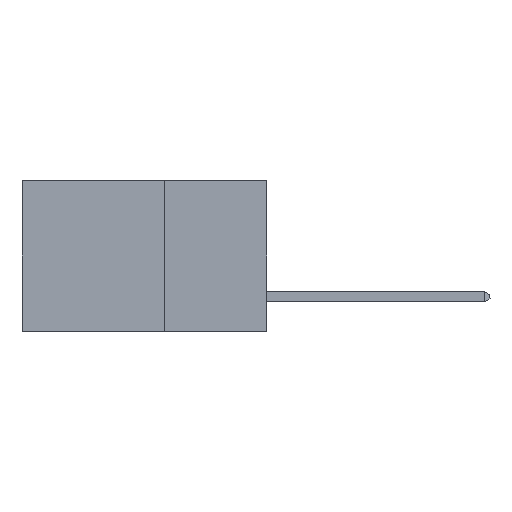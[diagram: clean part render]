
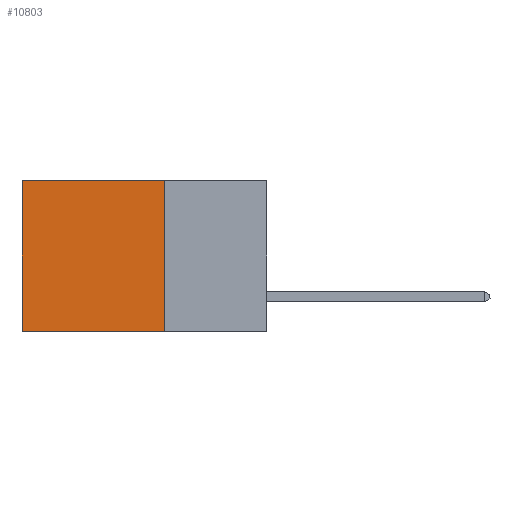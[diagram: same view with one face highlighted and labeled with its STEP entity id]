
A CAD part, left-side view. The second image highlights one B-rep face of the part: STEP entity #10803.
In plain terms, the highlighted planar face has unit normal (-1, 0, 0).
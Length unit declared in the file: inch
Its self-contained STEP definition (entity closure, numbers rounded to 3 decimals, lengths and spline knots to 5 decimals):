
#1214 = DIRECTION ( 'NONE',  ( 1., 0., 0. ) ) ;
#2312 = DIRECTION ( 'NONE',  ( 0., 0., -1. ) ) ;
#2350 = DIRECTION ( 'NONE',  ( 0., 1., 0. ) ) ;
#3029 = ORIENTED_EDGE ( 'NONE', *, *, #13267, .T. ) ;
#4931 = PLANE ( 'NONE',  #16104 ) ;
#4991 = LINE ( 'NONE', #15347, #39008 ) ;
#9588 = VECTOR ( 'NONE', #19865, 39.37008 ) ;
#10803 = ADVANCED_FACE ( 'NONE', ( #30011 ), #4931, .F. ) ;
#11649 = CARTESIAN_POINT ( 'NONE',  ( 0.2875, 0.25, 0. ) ) ;
#11871 = EDGE_LOOP ( 'NONE', ( #3029, #21379, #25683, #42463 ) ) ;
#13094 = CARTESIAN_POINT ( 'NONE',  ( 0.2875, 0.25, 0. ) ) ;
#13267 = EDGE_CURVE ( 'NONE', #24993, #21415, #4991, .T. ) ;
#14691 = LINE ( 'NONE', #28683, #17272 ) ;
#14811 = CARTESIAN_POINT ( 'NONE',  ( 0.2875, 0.25, 0. ) ) ;
#15260 = CARTESIAN_POINT ( 'NONE',  ( 0.2875, 0.6, 0. ) ) ;
#15303 = VERTEX_POINT ( 'NONE', #42365 ) ;
#15347 = CARTESIAN_POINT ( 'NONE',  ( 0.2875, 0.6, 0. ) ) ;
#16104 = AXIS2_PLACEMENT_3D ( 'NONE', #14811, #1214, #41084 ) ;
#17272 = VECTOR ( 'NONE', #2350, 39.37008 ) ;
#19865 = DIRECTION ( 'NONE',  ( 0., 0., -1. ) ) ;
#21379 = ORIENTED_EDGE ( 'NONE', *, *, #32803, .F. ) ;
#21415 = VERTEX_POINT ( 'NONE', #30343 ) ;
#24993 = VERTEX_POINT ( 'NONE', #15260 ) ;
#25220 = VECTOR ( 'NONE', #31763, 39.37008 ) ;
#25683 = ORIENTED_EDGE ( 'NONE', *, *, #28524, .F. ) ;
#28524 = EDGE_CURVE ( 'NONE', #15303, #42209, #40063, .T. ) ;
#28683 = CARTESIAN_POINT ( 'NONE',  ( 0.2875, 0.25, -0.37 ) ) ;
#30011 = FACE_OUTER_BOUND ( 'NONE', #11871, .T. ) ;
#30343 = CARTESIAN_POINT ( 'NONE',  ( 0.2875, 0.6, -0.37 ) ) ;
#31763 = DIRECTION ( 'NONE',  ( 0., 1., 0. ) ) ;
#32803 = EDGE_CURVE ( 'NONE', #42209, #21415, #14691, .T. ) ;
#34030 = LINE ( 'NONE', #11649, #25220 ) ;
#36169 = EDGE_CURVE ( 'NONE', #15303, #24993, #34030, .T. ) ;
#38976 = CARTESIAN_POINT ( 'NONE',  ( 0.2875, 0.25, -0.37 ) ) ;
#39008 = VECTOR ( 'NONE', #2312, 39.37008 ) ;
#40063 = LINE ( 'NONE', #13094, #9588 ) ;
#41084 = DIRECTION ( 'NONE',  ( 0., 0., -1. ) ) ;
#42209 = VERTEX_POINT ( 'NONE', #38976 ) ;
#42365 = CARTESIAN_POINT ( 'NONE',  ( 0.2875, 0.25, 0. ) ) ;
#42463 = ORIENTED_EDGE ( 'NONE', *, *, #36169, .T. ) ;
